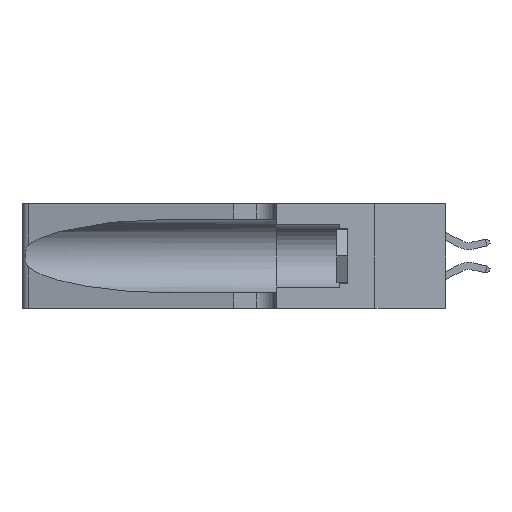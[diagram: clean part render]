
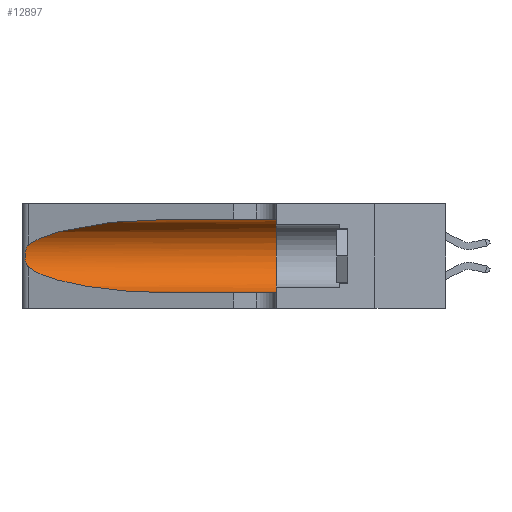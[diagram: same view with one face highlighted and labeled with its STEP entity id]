
A CAD part, left-side view. The second image highlights one B-rep face of the part: STEP entity #12897.
In plain terms, the highlighted cylindrical face has radius 3.308 mm (diameter 6.617 mm), a partial arc.
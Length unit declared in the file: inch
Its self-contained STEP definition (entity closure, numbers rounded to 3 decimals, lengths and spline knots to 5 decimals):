
#401 = AXIS2_PLACEMENT_3D ( 'NONE', #6117, #30172, #9582 ) ;
#480 = VERTEX_POINT ( 'NONE', #26176 ) ;
#654 = VERTEX_POINT ( 'NONE', #27048 ) ;
#841 = CARTESIAN_POINT ( 'NONE',  ( 0.18966, 0.96281, 0.05475 ) ) ;
#1066 = CARTESIAN_POINT ( 'NONE',  ( 0.25854, 1.2359, 0.20912 ) ) ;
#2090 = CARTESIAN_POINT ( 'NONE',  ( 0.1305, 0.72297, 0.31525 ) ) ;
#2215 = VERTEX_POINT ( 'NONE', #42082 ) ;
#2222 = EDGE_CURVE ( 'NONE', #654, #480, #25615, .T. ) ;
#2445 = VERTEX_POINT ( 'NONE', #26367 ) ;
#2565 = EDGE_CURVE ( 'NONE', #2215, #42046, #6016, .T. ) ;
#2892 = EDGE_CURVE ( 'NONE', #2445, #4688, #37641, .T. ) ;
#4558 = CARTESIAN_POINT ( 'NONE',  ( 0.26075, 1.23896, 0.19203 ) ) ;
#4688 = VERTEX_POINT ( 'NONE', #24565 ) ;
#4882 = VECTOR ( 'NONE', #26950, 39.37008 ) ;
#5405 = EDGE_LOOP ( 'NONE', ( #28139, #43962, #38254, #28176, #34706, #9678 ) ) ;
#6016 = LINE ( 'NONE', #9751, #4882 ) ;
#6117 = CARTESIAN_POINT ( 'NONE',  ( 0.1305, 0.35, 0.185 ) ) ;
#8078 = CARTESIAN_POINT ( 'NONE',  ( 0.26017, 1.23833, 0.17102 ) ) ;
#9091 = CARTESIAN_POINT ( 'NONE',  ( 0.2373, 1.15595, 0.28018 ) ) ;
#9582 = DIRECTION ( 'NONE',  ( 0., 0., 1. ) ) ;
#9678 = ORIENTED_EDGE ( 'NONE', *, *, #2565, .F. ) ;
#9751 = CARTESIAN_POINT ( 'NONE',  ( 0.1305, 1.61858, 0.31525 ) ) ;
#10927 =( BOUNDED_CURVE ( )  B_SPLINE_CURVE ( 3, ( #2090, #36382, #9091, #33135 ),
 .UNSPECIFIED., .F., .T. ) 
 B_SPLINE_CURVE_WITH_KNOTS ( ( 4, 4 ),
 ( 1.5708, 2.84003 ),
 .UNSPECIFIED. ) 
 CURVE ( )  GEOMETRIC_REPRESENTATION_ITEM ( )  RATIONAL_B_SPLINE_CURVE ( ( 1., 0.87, 0.87, 1. ) ) 
 REPRESENTATION_ITEM ( '' )  );
#11392 = CARTESIAN_POINT ( 'NONE',  ( 0.25555, 1.22994, 0.2215 ) ) ;
#11529 = CARTESIAN_POINT ( 'NONE',  ( 0.25789, 1.23486, 0.15765 ) ) ;
#12897 = ADVANCED_FACE ( 'NONE', ( #14186 ), #39363, .F. ) ;
#14186 = FACE_OUTER_BOUND ( 'NONE', #5405, .T. ) ;
#14345 = DIRECTION ( 'NONE',  ( 0., 0., -1. ) ) ;
#15010 = CARTESIAN_POINT ( 'NONE',  ( 0.25555, 1.22993, 0.14849 ) ) ;
#18147 = CARTESIAN_POINT ( 'NONE',  ( 0.25487, 1.22718, 0.14631 ) ) ;
#18977 = CARTESIAN_POINT ( 'NONE',  ( 0.1305, 1.61858, 0.05475 ) ) ;
#21846 = CARTESIAN_POINT ( 'NONE',  ( 0.25787, 1.23484, 0.2124 ) ) ;
#22318 =( BOUNDED_CURVE ( )  B_SPLINE_CURVE ( 3, ( #18147, #38575, #841, #25063 ),
 .UNSPECIFIED., .F., .T. ) 
 B_SPLINE_CURVE_WITH_KNOTS ( ( 4, 4 ),
 ( 3.44316, 4.71239 ),
 .UNSPECIFIED. ) 
 CURVE ( )  GEOMETRIC_REPRESENTATION_ITEM ( )  RATIONAL_B_SPLINE_CURVE ( ( 1., 0.87, 0.87, 1. ) ) 
 REPRESENTATION_ITEM ( '' )  );
#24565 = CARTESIAN_POINT ( 'NONE',  ( 0.1305, 0.35, 0.05475 ) ) ;
#24804 = CARTESIAN_POINT ( 'NONE',  ( 0.1305, 1.61858, 0.185 ) ) ;
#25063 = CARTESIAN_POINT ( 'NONE',  ( 0.1305, 0.72297, 0.05475 ) ) ;
#25295 = CARTESIAN_POINT ( 'NONE',  ( 0.26018, 1.23835, 0.19895 ) ) ;
#25615 = B_SPLINE_CURVE_WITH_KNOTS ( 'NONE', 3,
 ( #38802, #11392, #42232, #21846, #1066, #25295, #4558, #28677, #8078, #32109, #11529, #35522, #15010, #38950 ),
 .UNSPECIFIED., .F., .F.,
 ( 4, 2, 2, 2, 2, 2, 4 ),
 ( 0., 0.00027, 0.00053, 0.00107, 0.0016, 0.00187, 0.00214 ),
 .UNSPECIFIED. ) ;
#25788 = EDGE_CURVE ( 'NONE', #480, #2445, #22318, .T. ) ;
#26176 = CARTESIAN_POINT ( 'NONE',  ( 0.25487, 1.22718, 0.14631 ) ) ;
#26367 = CARTESIAN_POINT ( 'NONE',  ( 0.1305, 0.72297, 0.05475 ) ) ;
#26950 = DIRECTION ( 'NONE',  ( 0., -1., 0. ) ) ;
#27048 = CARTESIAN_POINT ( 'NONE',  ( 0.25487, 1.22718, 0.22369 ) ) ;
#28139 = ORIENTED_EDGE ( 'NONE', *, *, #41008, .T. ) ;
#28176 = ORIENTED_EDGE ( 'NONE', *, *, #2892, .T. ) ;
#28194 = DIRECTION ( 'NONE',  ( 0., -1., 0. ) ) ;
#28677 = CARTESIAN_POINT ( 'NONE',  ( 0.26075, 1.23896, 0.178 ) ) ;
#28881 = CIRCLE ( 'NONE', #401, 0.13025 ) ;
#29325 = EDGE_CURVE ( 'NONE', #42046, #4688, #28881, .T. ) ;
#30172 = DIRECTION ( 'NONE',  ( 0., 1., 0. ) ) ;
#32109 = CARTESIAN_POINT ( 'NONE',  ( 0.25856, 1.23593, 0.16098 ) ) ;
#33135 = CARTESIAN_POINT ( 'NONE',  ( 0.25487, 1.22718, 0.22369 ) ) ;
#34706 = ORIENTED_EDGE ( 'NONE', *, *, #29325, .F. ) ;
#35522 = CARTESIAN_POINT ( 'NONE',  ( 0.25639, 1.23186, 0.15144 ) ) ;
#36382 = CARTESIAN_POINT ( 'NONE',  ( 0.18966, 0.96281, 0.31525 ) ) ;
#36576 = VECTOR ( 'NONE', #39243, 39.37008 ) ;
#37641 = LINE ( 'NONE', #18977, #36576 ) ;
#38254 = ORIENTED_EDGE ( 'NONE', *, *, #25788, .T. ) ;
#38575 = CARTESIAN_POINT ( 'NONE',  ( 0.2373, 1.15595, 0.08982 ) ) ;
#38802 = CARTESIAN_POINT ( 'NONE',  ( 0.25487, 1.22718, 0.22369 ) ) ;
#38950 = CARTESIAN_POINT ( 'NONE',  ( 0.25487, 1.22718, 0.14631 ) ) ;
#39243 = DIRECTION ( 'NONE',  ( 0., -1., 0. ) ) ;
#39363 = CYLINDRICAL_SURFACE ( 'NONE', #43154, 0.13025 ) ;
#41008 = EDGE_CURVE ( 'NONE', #2215, #654, #10927, .T. ) ;
#41525 = CARTESIAN_POINT ( 'NONE',  ( 0.1305, 0.35, 0.31525 ) ) ;
#42046 = VERTEX_POINT ( 'NONE', #41525 ) ;
#42082 = CARTESIAN_POINT ( 'NONE',  ( 0.1305, 0.72297, 0.31525 ) ) ;
#42232 = CARTESIAN_POINT ( 'NONE',  ( 0.25639, 1.23184, 0.21858 ) ) ;
#43154 = AXIS2_PLACEMENT_3D ( 'NONE', #24804, #28194, #14345 ) ;
#43962 = ORIENTED_EDGE ( 'NONE', *, *, #2222, .T. ) ;
